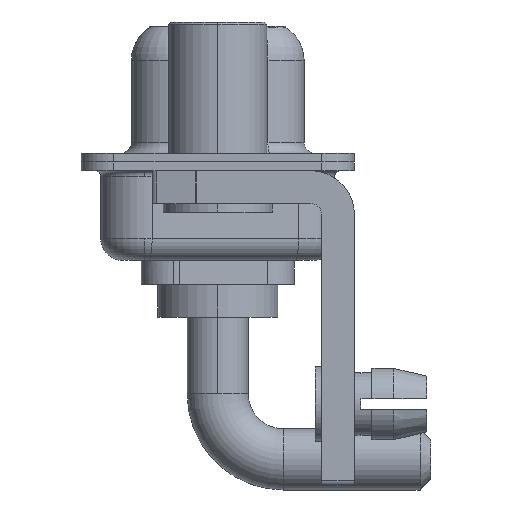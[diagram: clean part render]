
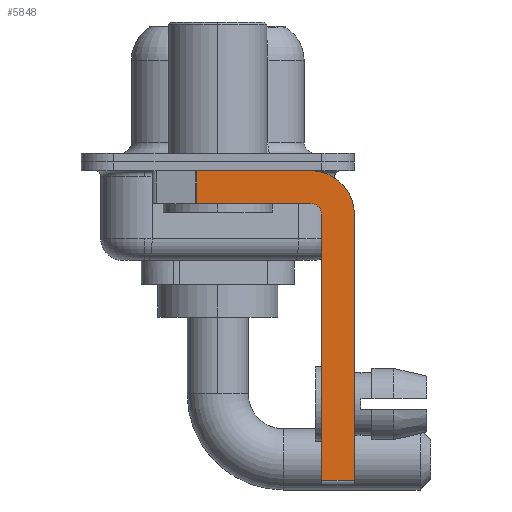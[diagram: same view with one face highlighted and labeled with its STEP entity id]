
A CAD part, left-side view. The second image highlights one B-rep face of the part: STEP entity #5848.
In plain terms, the highlighted planar face has unit normal (-1, 0, 0).
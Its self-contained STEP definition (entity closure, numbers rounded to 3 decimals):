
#249 = DIRECTION ( 'NONE',  ( -1., 0., 0. ) ) ;
#277 = EDGE_CURVE ( 'NONE', #420, #5424, #6703, .T. ) ;
#293 = CARTESIAN_POINT ( 'NONE',  ( -2.9, -4.25, -1.9 ) ) ;
#322 = LINE ( 'NONE', #6284, #3160 ) ;
#420 = VERTEX_POINT ( 'NONE', #5898 ) ;
#561 = PLANE ( 'NONE',  #13453 ) ;
#1529 = VERTEX_POINT ( 'NONE', #10524 ) ;
#1534 = LINE ( 'NONE', #6453, #4630 ) ;
#1625 = DIRECTION ( 'NONE',  ( 1., 0., 0. ) ) ;
#1706 = DIRECTION ( 'NONE',  ( 0., 0., -1. ) ) ;
#1891 = EDGE_CURVE ( 'NONE', #13132, #6410, #8979, .T. ) ;
#1920 = CARTESIAN_POINT ( 'NONE',  ( -2.9, -4.75, -14.55 ) ) ;
#2006 = DIRECTION ( 'NONE',  ( 0., 0., -1. ) ) ;
#3084 = LINE ( 'NONE', #15210, #6180 ) ;
#3105 = ORIENTED_EDGE ( 'NONE', *, *, #10648, .F. ) ;
#3160 = VECTOR ( 'NONE', #13755, 1000. ) ;
#3364 = CARTESIAN_POINT ( 'NONE',  ( -2.9, -4.75, -2.4 ) ) ;
#3391 = CIRCLE ( 'NONE', #14679, 2. ) ;
#4064 = VECTOR ( 'NONE', #13058, 1000. ) ;
#4346 = ORIENTED_EDGE ( 'NONE', *, *, #8271, .F. ) ;
#4350 = LINE ( 'NONE', #12953, #4643 ) ;
#4630 = VECTOR ( 'NONE', #12330, 1000. ) ;
#4643 = VECTOR ( 'NONE', #14151, 1000. ) ;
#4756 = VERTEX_POINT ( 'NONE', #293 ) ;
#4844 = AXIS2_PLACEMENT_3D ( 'NONE', #8953, #249, #5328 ) ;
#5152 = EDGE_CURVE ( 'NONE', #6410, #4756, #5604, .T. ) ;
#5328 = DIRECTION ( 'NONE',  ( 0., 0., 1. ) ) ;
#5424 = VERTEX_POINT ( 'NONE', #9121 ) ;
#5604 = CIRCLE ( 'NONE', #4844, 0.5 ) ;
#5641 = ORIENTED_EDGE ( 'NONE', *, *, #1891, .F. ) ;
#5764 = ORIENTED_EDGE ( 'NONE', *, *, #5152, .F. ) ;
#5848 = ADVANCED_FACE ( 'NONE', ( #7886 ), #561, .F. ) ;
#5898 = CARTESIAN_POINT ( 'NONE',  ( -2.9, -6.25, -2.4 ) ) ;
#6002 = CARTESIAN_POINT ( 'NONE',  ( -2.9, 0.978, -0.4 ) ) ;
#6180 = VECTOR ( 'NONE', #11596, 1000. ) ;
#6284 = CARTESIAN_POINT ( 'NONE',  ( -2.9, -4.25, -14.55 ) ) ;
#6410 = VERTEX_POINT ( 'NONE', #3364 ) ;
#6453 = CARTESIAN_POINT ( 'NONE',  ( -2.9, -4.25, -1.9 ) ) ;
#6703 = LINE ( 'NONE', #8154, #4064 ) ;
#7472 = VERTEX_POINT ( 'NONE', #13815 ) ;
#7766 = ORIENTED_EDGE ( 'NONE', *, *, #9811, .F. ) ;
#7886 = FACE_OUTER_BOUND ( 'NONE', #10550, .T. ) ;
#8154 = CARTESIAN_POINT ( 'NONE',  ( -2.9, -6.25, -2.4 ) ) ;
#8271 = EDGE_CURVE ( 'NONE', #4756, #1529, #1534, .T. ) ;
#8361 = EDGE_CURVE ( 'NONE', #12989, #1529, #3084, .T. ) ;
#8818 = ORIENTED_EDGE ( 'NONE', *, *, #8361, .T. ) ;
#8953 = CARTESIAN_POINT ( 'NONE',  ( -2.9, -4.25, -2.4 ) ) ;
#8979 = LINE ( 'NONE', #12829, #15615 ) ;
#9121 = CARTESIAN_POINT ( 'NONE',  ( -2.9, -6.25, -14.55 ) ) ;
#9811 = EDGE_CURVE ( 'NONE', #12989, #7472, #4350, .T. ) ;
#10524 = CARTESIAN_POINT ( 'NONE',  ( -2.9, 0.978, -1.9 ) ) ;
#10550 = EDGE_LOOP ( 'NONE', ( #7766, #8818, #4346, #5764, #5641, #12947, #15805, #3105 ) ) ;
#10648 = EDGE_CURVE ( 'NONE', #7472, #420, #3391, .T. ) ;
#11596 = DIRECTION ( 'NONE',  ( 0., 0., -1. ) ) ;
#11599 = EDGE_CURVE ( 'NONE', #13132, #5424, #322, .T. ) ;
#11661 = CARTESIAN_POINT ( 'NONE',  ( -2.9, -4.25, -2.4 ) ) ;
#11815 = DIRECTION ( 'NONE',  ( 1., 0., 0. ) ) ;
#12330 = DIRECTION ( 'NONE',  ( 0., 1., 0. ) ) ;
#12491 = CARTESIAN_POINT ( 'NONE',  ( -2.9, -4.25, -2.4 ) ) ;
#12829 = CARTESIAN_POINT ( 'NONE',  ( -2.9, -4.75, -14.8 ) ) ;
#12947 = ORIENTED_EDGE ( 'NONE', *, *, #11599, .T. ) ;
#12953 = CARTESIAN_POINT ( 'NONE',  ( -2.9, 3., -0.4 ) ) ;
#12989 = VERTEX_POINT ( 'NONE', #6002 ) ;
#13058 = DIRECTION ( 'NONE',  ( 0., 0., -1. ) ) ;
#13132 = VERTEX_POINT ( 'NONE', #1920 ) ;
#13453 = AXIS2_PLACEMENT_3D ( 'NONE', #11661, #11815, #2006 ) ;
#13755 = DIRECTION ( 'NONE',  ( 0., -1., 0. ) ) ;
#13815 = CARTESIAN_POINT ( 'NONE',  ( -2.9, -4.25, -0.4 ) ) ;
#13873 = DIRECTION ( 'NONE',  ( 0., 0., 1. ) ) ;
#14151 = DIRECTION ( 'NONE',  ( 0., -1., 0. ) ) ;
#14679 = AXIS2_PLACEMENT_3D ( 'NONE', #12491, #1625, #1706 ) ;
#15210 = CARTESIAN_POINT ( 'NONE',  ( -2.9, 0.978, -1.9 ) ) ;
#15615 = VECTOR ( 'NONE', #13873, 1000. ) ;
#15805 = ORIENTED_EDGE ( 'NONE', *, *, #277, .F. ) ;
